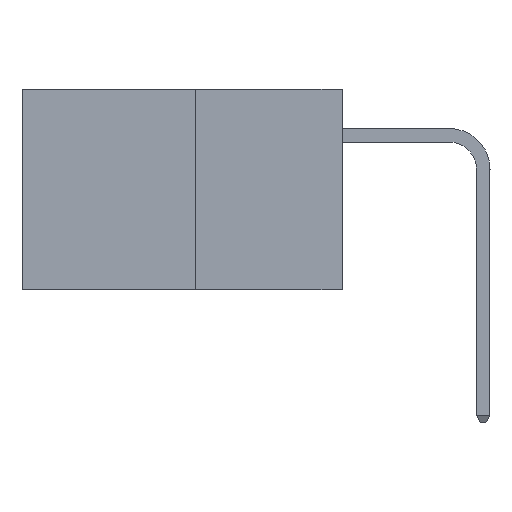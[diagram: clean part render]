
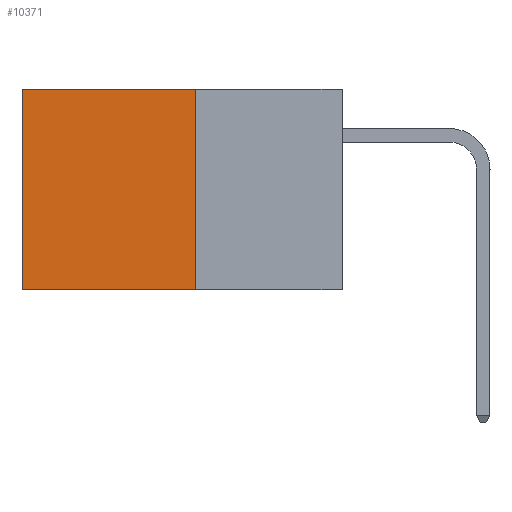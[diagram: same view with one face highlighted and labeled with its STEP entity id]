
A CAD part, left-side view. The second image highlights one B-rep face of the part: STEP entity #10371.
In plain terms, the highlighted planar face has unit normal (-1, 0, 0).
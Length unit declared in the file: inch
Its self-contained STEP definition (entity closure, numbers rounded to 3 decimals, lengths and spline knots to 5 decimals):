
#116 = DIRECTION ( 'NONE',  ( 0., 1., 0. ) ) ;
#1167 = EDGE_CURVE ( 'NONE', #5054, #3217, #5358, .T. ) ;
#1619 = CARTESIAN_POINT ( 'NONE',  ( 0.277, 0.59, -0.37 ) ) ;
#2156 = EDGE_CURVE ( 'NONE', #7372, #3217, #4340, .T. ) ;
#2605 = CARTESIAN_POINT ( 'NONE',  ( 0.277, 0.59, -0.37 ) ) ;
#3217 = VERTEX_POINT ( 'NONE', #1619 ) ;
#3596 = LINE ( 'NONE', #9449, #11634 ) ;
#3825 = ORIENTED_EDGE ( 'NONE', *, *, #4951, .T. ) ;
#3989 = EDGE_CURVE ( 'NONE', #13727, #7372, #3596, .T. ) ;
#4340 = LINE ( 'NONE', #7164, #6459 ) ;
#4903 = CARTESIAN_POINT ( 'NONE',  ( 0.277, 0.59, 0. ) ) ;
#4951 = EDGE_CURVE ( 'NONE', #13727, #5054, #6406, .T. ) ;
#5018 = VECTOR ( 'NONE', #7956, 39.37008 ) ;
#5054 = VERTEX_POINT ( 'NONE', #4903 ) ;
#5358 = LINE ( 'NONE', #2605, #5018 ) ;
#5590 = DIRECTION ( 'NONE',  ( 0., 0., -1. ) ) ;
#5608 = DIRECTION ( 'NONE',  ( 1., 0., 0. ) ) ;
#5622 = PLANE ( 'NONE',  #12328 ) ;
#5662 = CARTESIAN_POINT ( 'NONE',  ( 0.277, 0.27, -0.37 ) ) ;
#6082 = VECTOR ( 'NONE', #7992, 39.37008 ) ;
#6301 = ORIENTED_EDGE ( 'NONE', *, *, #2156, .F. ) ;
#6406 = LINE ( 'NONE', #8192, #6082 ) ;
#6459 = VECTOR ( 'NONE', #116, 39.37008 ) ;
#7164 = CARTESIAN_POINT ( 'NONE',  ( 0.277, 0.27, -0.37 ) ) ;
#7372 = VERTEX_POINT ( 'NONE', #11652 ) ;
#7956 = DIRECTION ( 'NONE',  ( 0., 0., -1. ) ) ;
#7992 = DIRECTION ( 'NONE',  ( 0., 1., 0. ) ) ;
#8192 = CARTESIAN_POINT ( 'NONE',  ( 0.277, 0.27, 0. ) ) ;
#8756 = ORIENTED_EDGE ( 'NONE', *, *, #1167, .T. ) ;
#8841 = DIRECTION ( 'NONE',  ( 0., 0., -1. ) ) ;
#9067 = ORIENTED_EDGE ( 'NONE', *, *, #3989, .F. ) ;
#9449 = CARTESIAN_POINT ( 'NONE',  ( 0.277, 0.27, -0.37 ) ) ;
#9956 = EDGE_LOOP ( 'NONE', ( #8756, #6301, #9067, #3825 ) ) ;
#10371 = ADVANCED_FACE ( 'NONE', ( #11321 ), #5622, .F. ) ;
#11321 = FACE_OUTER_BOUND ( 'NONE', #9956, .T. ) ;
#11634 = VECTOR ( 'NONE', #8841, 39.37008 ) ;
#11652 = CARTESIAN_POINT ( 'NONE',  ( 0.277, 0.27, -0.37 ) ) ;
#12328 = AXIS2_PLACEMENT_3D ( 'NONE', #5662, #5608, #5590 ) ;
#13028 = CARTESIAN_POINT ( 'NONE',  ( 0.277, 0.27, 0. ) ) ;
#13727 = VERTEX_POINT ( 'NONE', #13028 ) ;
